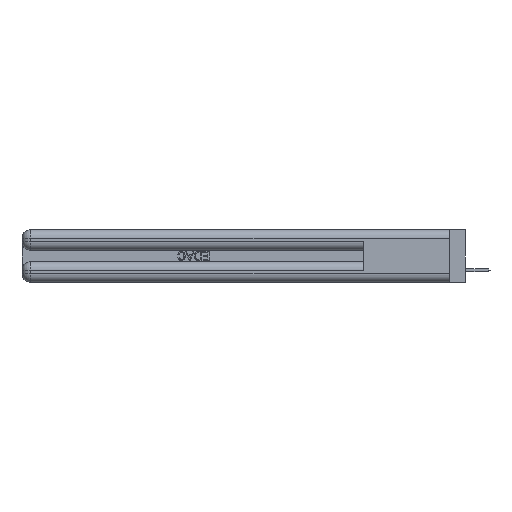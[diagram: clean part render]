
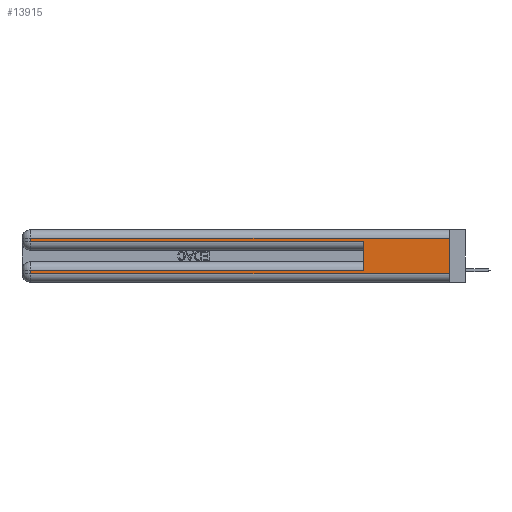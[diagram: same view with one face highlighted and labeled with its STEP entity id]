
A CAD part, left-side view. The second image highlights one B-rep face of the part: STEP entity #13915.
In plain terms, the highlighted planar face has unit normal (-1, 0, 0).
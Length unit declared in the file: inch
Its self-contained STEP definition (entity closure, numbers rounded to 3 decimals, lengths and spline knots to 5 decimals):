
#350 = VERTEX_POINT ( 'NONE', #15587 ) ;
#376 = LINE ( 'NONE', #25813, #29117 ) ;
#980 = CARTESIAN_POINT ( 'NONE',  ( 0., 2.94, 0.085 ) ) ;
#1760 = CARTESIAN_POINT ( 'NONE',  ( 0., 2.94, 0.37 ) ) ;
#2061 = CARTESIAN_POINT ( 'NONE',  ( 0., 0., 0.085 ) ) ;
#2188 = DIRECTION ( 'NONE',  ( 0., 0., 1. ) ) ;
#2380 = DIRECTION ( 'NONE',  ( 0., 1., 0. ) ) ;
#2509 = ORIENTED_EDGE ( 'NONE', *, *, #43233, .T. ) ;
#4104 = AXIS2_PLACEMENT_3D ( 'NONE', #31802, #14682, #11210 ) ;
#5550 = CARTESIAN_POINT ( 'NONE',  ( 0., 2.94, 0.06 ) ) ;
#6130 = VERTEX_POINT ( 'NONE', #980 ) ;
#6146 = ORIENTED_EDGE ( 'NONE', *, *, #34699, .T. ) ;
#7238 = CARTESIAN_POINT ( 'NONE',  ( 0., 0.6, 0.285 ) ) ;
#7595 = ORIENTED_EDGE ( 'NONE', *, *, #14220, .T. ) ;
#8780 = DIRECTION ( 'NONE',  ( 0., 1., 0. ) ) ;
#9081 = CARTESIAN_POINT ( 'NONE',  ( 0., 0.6, 0.145 ) ) ;
#9779 = LINE ( 'NONE', #1760, #36896 ) ;
#11210 = DIRECTION ( 'NONE',  ( 0., 0., -1. ) ) ;
#12720 = VERTEX_POINT ( 'NONE', #21900 ) ;
#13915 = ADVANCED_FACE ( 'NONE', ( #32590 ), #31373, .F. ) ;
#13926 = VERTEX_POINT ( 'NONE', #25419 ) ;
#14211 = LINE ( 'NONE', #2061, #44737 ) ;
#14220 = EDGE_CURVE ( 'NONE', #6130, #26833, #17952, .T. ) ;
#14679 = VECTOR ( 'NONE', #16180, 39.37008 ) ;
#14682 = DIRECTION ( 'NONE',  ( 1., 0., 0. ) ) ;
#15587 = CARTESIAN_POINT ( 'NONE',  ( 0., 0., 0.06 ) ) ;
#16028 = CARTESIAN_POINT ( 'NONE',  ( 0., 2.94, 0.37 ) ) ;
#16180 = DIRECTION ( 'NONE',  ( 0., 0., -1. ) ) ;
#16541 = ORIENTED_EDGE ( 'NONE', *, *, #40044, .F. ) ;
#17952 = LINE ( 'NONE', #16028, #14679 ) ;
#18076 = VERTEX_POINT ( 'NONE', #40928 ) ;
#18319 = VECTOR ( 'NONE', #40555, 39.37008 ) ;
#18450 = EDGE_CURVE ( 'NONE', #26833, #350, #25351, .T. ) ;
#19564 = EDGE_CURVE ( 'NONE', #18076, #40819, #45026, .T. ) ;
#21900 = CARTESIAN_POINT ( 'NONE',  ( 0., 2.94, 0.31 ) ) ;
#22113 = ORIENTED_EDGE ( 'NONE', *, *, #18450, .T. ) ;
#23800 = ORIENTED_EDGE ( 'NONE', *, *, #19564, .F. ) ;
#23909 = DIRECTION ( 'NONE',  ( 0., -1., 0. ) ) ;
#24300 = ORIENTED_EDGE ( 'NONE', *, *, #39482, .T. ) ;
#25351 = LINE ( 'NONE', #40406, #18319 ) ;
#25419 = CARTESIAN_POINT ( 'NONE',  ( 0., 0., 0.31 ) ) ;
#25813 = CARTESIAN_POINT ( 'NONE',  ( 0., 0., 0.37 ) ) ;
#26148 = EDGE_LOOP ( 'NONE', ( #16541, #24300, #2509, #6146, #23800, #30258, #7595, #22113 ) ) ;
#26833 = VERTEX_POINT ( 'NONE', #5550 ) ;
#27150 = LINE ( 'NONE', #41565, #34240 ) ;
#29117 = VECTOR ( 'NONE', #32789, 39.37008 ) ;
#29823 = VERTEX_POINT ( 'NONE', #42295 ) ;
#30258 = ORIENTED_EDGE ( 'NONE', *, *, #37721, .T. ) ;
#31373 = PLANE ( 'NONE',  #4104 ) ;
#31802 = CARTESIAN_POINT ( 'NONE',  ( 0., 0., 0.37 ) ) ;
#32590 = FACE_OUTER_BOUND ( 'NONE', #26148, .T. ) ;
#32789 = DIRECTION ( 'NONE',  ( 0., 0., -1. ) ) ;
#33014 = LINE ( 'NONE', #37452, #37998 ) ;
#34240 = VECTOR ( 'NONE', #23909, 39.37008 ) ;
#34699 = EDGE_CURVE ( 'NONE', #29823, #40819, #27150, .T. ) ;
#36863 = DIRECTION ( 'NONE',  ( 0., 0., -1. ) ) ;
#36896 = VECTOR ( 'NONE', #36863, 39.37008 ) ;
#37452 = CARTESIAN_POINT ( 'NONE',  ( 0., 0., 0.31 ) ) ;
#37721 = EDGE_CURVE ( 'NONE', #18076, #6130, #14211, .T. ) ;
#37998 = VECTOR ( 'NONE', #2380, 39.37008 ) ;
#39482 = EDGE_CURVE ( 'NONE', #13926, #12720, #33014, .T. ) ;
#40044 = EDGE_CURVE ( 'NONE', #13926, #350, #376, .T. ) ;
#40406 = CARTESIAN_POINT ( 'NONE',  ( 0., 0., 0.06 ) ) ;
#40555 = DIRECTION ( 'NONE',  ( 0., -1., 0. ) ) ;
#40819 = VERTEX_POINT ( 'NONE', #7238 ) ;
#40928 = CARTESIAN_POINT ( 'NONE',  ( 0., 0.6, 0.085 ) ) ;
#41565 = CARTESIAN_POINT ( 'NONE',  ( 0., 0., 0.285 ) ) ;
#42295 = CARTESIAN_POINT ( 'NONE',  ( 0., 2.94, 0.285 ) ) ;
#43233 = EDGE_CURVE ( 'NONE', #12720, #29823, #9779, .T. ) ;
#44472 = VECTOR ( 'NONE', #2188, 39.37008 ) ;
#44737 = VECTOR ( 'NONE', #8780, 39.37008 ) ;
#45026 = LINE ( 'NONE', #9081, #44472 ) ;
